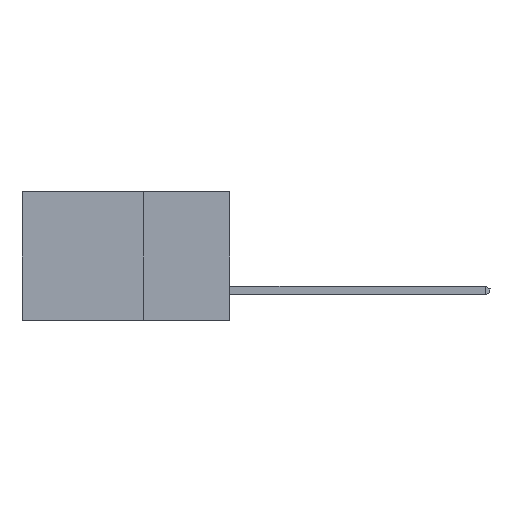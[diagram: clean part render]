
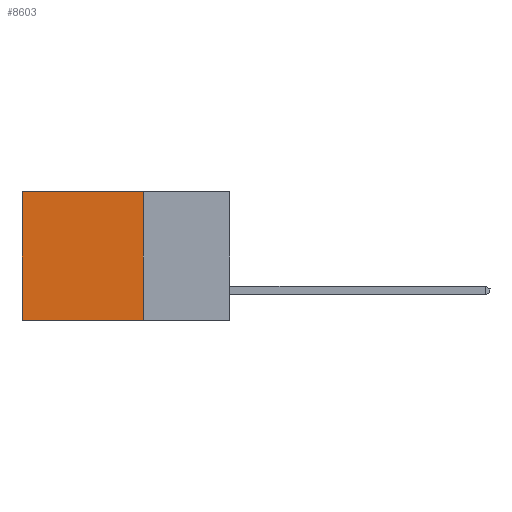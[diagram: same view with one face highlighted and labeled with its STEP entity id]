
A CAD part, left-side view. The second image highlights one B-rep face of the part: STEP entity #8603.
In plain terms, the highlighted planar face has unit normal (-1, 0, 0).
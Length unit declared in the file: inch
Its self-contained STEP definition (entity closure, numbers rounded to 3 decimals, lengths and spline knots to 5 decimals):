
#180 = EDGE_CURVE ( 'NONE', #9538, #4075, #5450, .T. ) ;
#1306 = DIRECTION ( 'NONE',  ( 0., 0., -1. ) ) ;
#2026 = VECTOR ( 'NONE', #5962, 39.37008 ) ;
#2077 = EDGE_CURVE ( 'NONE', #4075, #3487, #4751, .T. ) ;
#2326 = CARTESIAN_POINT ( 'NONE',  ( 0.2615, 0.25, -0.37 ) ) ;
#2436 = CARTESIAN_POINT ( 'NONE',  ( 0.2615, 0.25, -0.37 ) ) ;
#2664 = CARTESIAN_POINT ( 'NONE',  ( 0.2615, 0.25, 0. ) ) ;
#3010 = CARTESIAN_POINT ( 'NONE',  ( 0.2615, 0.6, -0.37 ) ) ;
#3182 = VECTOR ( 'NONE', #1306, 39.37008 ) ;
#3487 = VERTEX_POINT ( 'NONE', #8792 ) ;
#4075 = VERTEX_POINT ( 'NONE', #8142 ) ;
#4493 = ORIENTED_EDGE ( 'NONE', *, *, #2077, .T. ) ;
#4751 = LINE ( 'NONE', #3010, #3182 ) ;
#5039 = EDGE_CURVE ( 'NONE', #5650, #3487, #6645, .T. ) ;
#5450 = LINE ( 'NONE', #7104, #8710 ) ;
#5643 = VECTOR ( 'NONE', #10881, 39.37008 ) ;
#5650 = VERTEX_POINT ( 'NONE', #2436 ) ;
#5909 = DIRECTION ( 'NONE',  ( 0., 0., -1. ) ) ;
#5954 = PLANE ( 'NONE',  #7278 ) ;
#5962 = DIRECTION ( 'NONE',  ( 0., 1., 0. ) ) ;
#6355 = ORIENTED_EDGE ( 'NONE', *, *, #5039, .F. ) ;
#6513 = LINE ( 'NONE', #9971, #5643 ) ;
#6602 = ORIENTED_EDGE ( 'NONE', *, *, #180, .T. ) ;
#6645 = LINE ( 'NONE', #10106, #2026 ) ;
#7104 = CARTESIAN_POINT ( 'NONE',  ( 0.2615, 0.25, 0. ) ) ;
#7278 = AXIS2_PLACEMENT_3D ( 'NONE', #2326, #9293, #5909 ) ;
#8142 = CARTESIAN_POINT ( 'NONE',  ( 0.2615, 0.6, 0. ) ) ;
#8483 = EDGE_CURVE ( 'NONE', #9538, #5650, #6513, .T. ) ;
#8603 = ADVANCED_FACE ( 'NONE', ( #9226 ), #5954, .F. ) ;
#8710 = VECTOR ( 'NONE', #10723, 39.37008 ) ;
#8792 = CARTESIAN_POINT ( 'NONE',  ( 0.2615, 0.6, -0.37 ) ) ;
#9226 = FACE_OUTER_BOUND ( 'NONE', #10798, .T. ) ;
#9293 = DIRECTION ( 'NONE',  ( 1., 0., 0. ) ) ;
#9538 = VERTEX_POINT ( 'NONE', #2664 ) ;
#9971 = CARTESIAN_POINT ( 'NONE',  ( 0.2615, 0.25, -0.37 ) ) ;
#10104 = ORIENTED_EDGE ( 'NONE', *, *, #8483, .F. ) ;
#10106 = CARTESIAN_POINT ( 'NONE',  ( 0.2615, 0.25, -0.37 ) ) ;
#10723 = DIRECTION ( 'NONE',  ( 0., 1., 0. ) ) ;
#10798 = EDGE_LOOP ( 'NONE', ( #4493, #6355, #10104, #6602 ) ) ;
#10881 = DIRECTION ( 'NONE',  ( 0., 0., -1. ) ) ;
